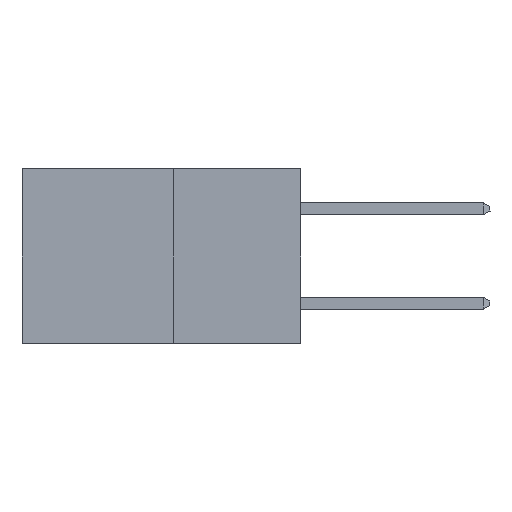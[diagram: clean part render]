
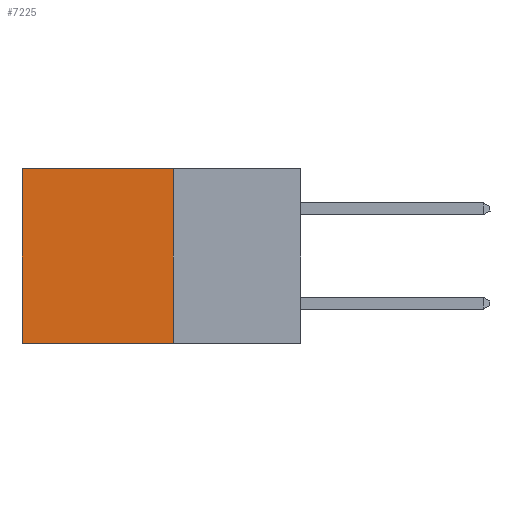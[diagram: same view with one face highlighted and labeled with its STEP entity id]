
A CAD part, left-side view. The second image highlights one B-rep face of the part: STEP entity #7225.
In plain terms, the highlighted planar face has unit normal (-1, 0, 0).
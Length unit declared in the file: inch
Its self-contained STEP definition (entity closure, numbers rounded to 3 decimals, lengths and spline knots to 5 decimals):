
#470 = VERTEX_POINT ( 'NONE', #25072 ) ;
#521 = VECTOR ( 'NONE', #3215, 39.37008 ) ;
#978 = CARTESIAN_POINT ( 'NONE',  ( 0.277, 0.27, -0.37 ) ) ;
#1110 = FACE_OUTER_BOUND ( 'NONE', #19269, .T. ) ;
#2816 = DIRECTION ( 'NONE',  ( 0., 0., -1. ) ) ;
#2913 = DIRECTION ( 'NONE',  ( 1., 0., 0. ) ) ;
#3166 = CARTESIAN_POINT ( 'NONE',  ( 0.277, 0.59, 0. ) ) ;
#3215 = DIRECTION ( 'NONE',  ( 0., 1., 0. ) ) ;
#4100 = EDGE_CURVE ( 'NONE', #470, #6615, #20928, .T. ) ;
#4339 = LINE ( 'NONE', #6179, #21856 ) ;
#4444 = DIRECTION ( 'NONE',  ( 0., 0., -1. ) ) ;
#4976 = ORIENTED_EDGE ( 'NONE', *, *, #4100, .F. ) ;
#5578 = CARTESIAN_POINT ( 'NONE',  ( 0.277, 0.27, -0.37 ) ) ;
#6179 = CARTESIAN_POINT ( 'NONE',  ( 0.277, 0.27, 0. ) ) ;
#6490 = CARTESIAN_POINT ( 'NONE',  ( 0.277, 0.27, -0.37 ) ) ;
#6615 = VERTEX_POINT ( 'NONE', #6490 ) ;
#7225 = ADVANCED_FACE ( 'NONE', ( #1110 ), #14581, .F. ) ;
#7795 = VERTEX_POINT ( 'NONE', #3166 ) ;
#8998 = ORIENTED_EDGE ( 'NONE', *, *, #9738, .F. ) ;
#9738 = EDGE_CURVE ( 'NONE', #6615, #23599, #17598, .T. ) ;
#10011 = AXIS2_PLACEMENT_3D ( 'NONE', #5578, #2913, #4444 ) ;
#11943 = CARTESIAN_POINT ( 'NONE',  ( 0.277, 0.59, -0.37 ) ) ;
#12898 = EDGE_CURVE ( 'NONE', #7795, #23599, #21039, .T. ) ;
#14581 = PLANE ( 'NONE',  #10011 ) ;
#14742 = VECTOR ( 'NONE', #2816, 39.37008 ) ;
#15315 = VECTOR ( 'NONE', #21457, 39.37008 ) ;
#17598 = LINE ( 'NONE', #978, #521 ) ;
#17612 = CARTESIAN_POINT ( 'NONE',  ( 0.277, 0.59, -0.37 ) ) ;
#17753 = CARTESIAN_POINT ( 'NONE',  ( 0.277, 0.27, -0.37 ) ) ;
#19269 = EDGE_LOOP ( 'NONE', ( #25284, #8998, #4976, #26058 ) ) ;
#20928 = LINE ( 'NONE', #17753, #15315 ) ;
#20940 = DIRECTION ( 'NONE',  ( 0., 1., 0. ) ) ;
#21039 = LINE ( 'NONE', #17612, #14742 ) ;
#21457 = DIRECTION ( 'NONE',  ( 0., 0., -1. ) ) ;
#21856 = VECTOR ( 'NONE', #20940, 39.37008 ) ;
#23599 = VERTEX_POINT ( 'NONE', #11943 ) ;
#24312 = EDGE_CURVE ( 'NONE', #470, #7795, #4339, .T. ) ;
#25072 = CARTESIAN_POINT ( 'NONE',  ( 0.277, 0.27, 0. ) ) ;
#25284 = ORIENTED_EDGE ( 'NONE', *, *, #12898, .T. ) ;
#26058 = ORIENTED_EDGE ( 'NONE', *, *, #24312, .T. ) ;
